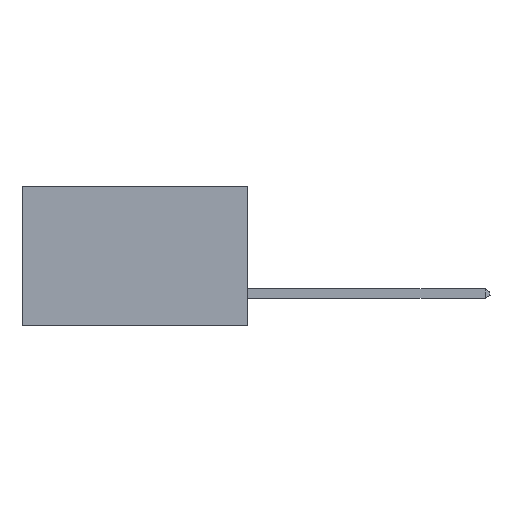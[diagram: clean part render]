
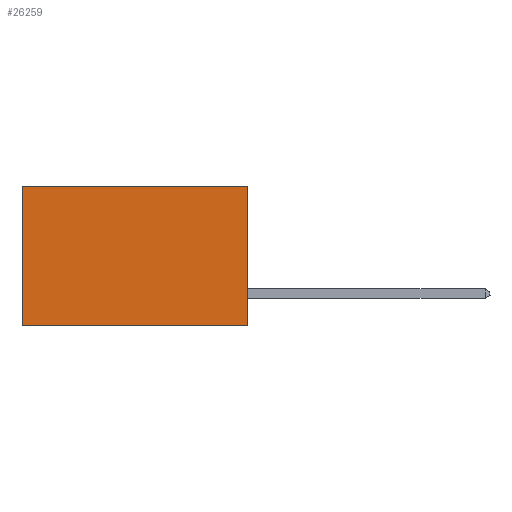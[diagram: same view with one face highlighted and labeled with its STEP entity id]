
A CAD part, left-side view. The second image highlights one B-rep face of the part: STEP entity #26259.
In plain terms, the highlighted planar face has unit normal (-1, 0, 0).
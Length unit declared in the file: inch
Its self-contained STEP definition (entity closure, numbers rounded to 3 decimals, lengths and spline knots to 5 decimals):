
#776 = CARTESIAN_POINT ( 'NONE',  ( 0.298, 0.6, 0. ) ) ;
#2260 = DIRECTION ( 'NONE',  ( 1., 0., 0. ) ) ;
#4950 = CARTESIAN_POINT ( 'NONE',  ( 0.298, 0., 0. ) ) ;
#5024 = PLANE ( 'NONE',  #8875 ) ;
#5132 = DIRECTION ( 'NONE',  ( 0., 0., -1. ) ) ;
#5926 = EDGE_CURVE ( 'NONE', #30912, #6268, #23080, .T. ) ;
#6268 = VERTEX_POINT ( 'NONE', #11710 ) ;
#6505 = DIRECTION ( 'NONE',  ( 0., 0., -1. ) ) ;
#7132 = EDGE_CURVE ( 'NONE', #20828, #6268, #18154, .T. ) ;
#8653 = DIRECTION ( 'NONE',  ( 0., 1., 0. ) ) ;
#8682 = VECTOR ( 'NONE', #8653, 39.37008 ) ;
#8754 = DIRECTION ( 'NONE',  ( 0., 1., 0. ) ) ;
#8875 = AXIS2_PLACEMENT_3D ( 'NONE', #9606, #2260, #5132 ) ;
#8896 = ORIENTED_EDGE ( 'NONE', *, *, #7132, .T. ) ;
#9606 = CARTESIAN_POINT ( 'NONE',  ( 0.298, 0., 0. ) ) ;
#11398 = EDGE_CURVE ( 'NONE', #11568, #20828, #12878, .T. ) ;
#11450 = EDGE_LOOP ( 'NONE', ( #8896, #17460, #20525, #20502 ) ) ;
#11568 = VERTEX_POINT ( 'NONE', #4950 ) ;
#11710 = CARTESIAN_POINT ( 'NONE',  ( 0.298, 0.6, -0.37 ) ) ;
#11770 = CARTESIAN_POINT ( 'NONE',  ( 0.298, 0., -0.37 ) ) ;
#12110 = DIRECTION ( 'NONE',  ( 0., 0., -1. ) ) ;
#12878 = LINE ( 'NONE', #20809, #8682 ) ;
#13580 = CARTESIAN_POINT ( 'NONE',  ( 0.298, 0., -0.37 ) ) ;
#16207 = VECTOR ( 'NONE', #6505, 39.37008 ) ;
#16221 = CARTESIAN_POINT ( 'NONE',  ( 0.298, 0.6, 0. ) ) ;
#17460 = ORIENTED_EDGE ( 'NONE', *, *, #5926, .F. ) ;
#18154 = LINE ( 'NONE', #16221, #16207 ) ;
#19878 = EDGE_CURVE ( 'NONE', #11568, #30912, #20346, .T. ) ;
#19944 = VECTOR ( 'NONE', #12110, 39.37008 ) ;
#20346 = LINE ( 'NONE', #24052, #19944 ) ;
#20502 = ORIENTED_EDGE ( 'NONE', *, *, #11398, .T. ) ;
#20525 = ORIENTED_EDGE ( 'NONE', *, *, #19878, .F. ) ;
#20809 = CARTESIAN_POINT ( 'NONE',  ( 0.298, 0., 0. ) ) ;
#20828 = VERTEX_POINT ( 'NONE', #776 ) ;
#23080 = LINE ( 'NONE', #13580, #24577 ) ;
#24052 = CARTESIAN_POINT ( 'NONE',  ( 0.298, 0., 0. ) ) ;
#24577 = VECTOR ( 'NONE', #8754, 39.37008 ) ;
#26259 = ADVANCED_FACE ( 'NONE', ( #29863 ), #5024, .F. ) ;
#29863 = FACE_OUTER_BOUND ( 'NONE', #11450, .T. ) ;
#30912 = VERTEX_POINT ( 'NONE', #11770 ) ;
